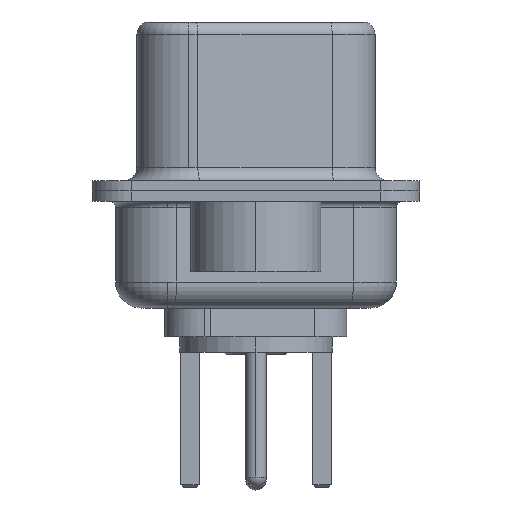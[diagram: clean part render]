
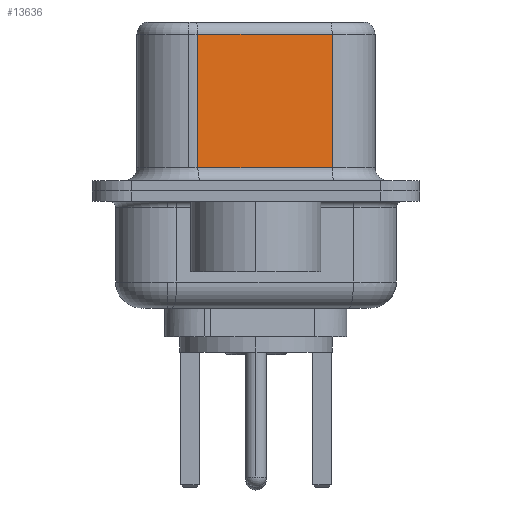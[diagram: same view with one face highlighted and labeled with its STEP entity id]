
A CAD part, left-side view. The second image highlights one B-rep face of the part: STEP entity #13636.
In plain terms, the highlighted planar face has unit normal (-0.985, -0.174, 0).
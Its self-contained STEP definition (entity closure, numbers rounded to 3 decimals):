
#1256 = VERTEX_POINT ( 'NONE', #13271 ) ;
#1541 = VECTOR ( 'NONE', #17890, 1000. ) ;
#1896 = DIRECTION ( 'NONE',  ( -0.174, 0.985, 0. ) ) ;
#2174 = EDGE_CURVE ( 'NONE', #6877, #3470, #17523, .T. ) ;
#2488 = EDGE_LOOP ( 'NONE', ( #5793, #9946, #18681, #13896 ) ) ;
#2517 = CARTESIAN_POINT ( 'NONE',  ( 4.565, -2.927, 6.02 ) ) ;
#3470 = VERTEX_POINT ( 'NONE', #10691 ) ;
#4288 = DIRECTION ( 'NONE',  ( 0., 0., -1. ) ) ;
#5793 = ORIENTED_EDGE ( 'NONE', *, *, #8785, .F. ) ;
#6603 = CARTESIAN_POINT ( 'NONE',  ( 4.565, -2.927, 6.02 ) ) ;
#6877 = VERTEX_POINT ( 'NONE', #15002 ) ;
#7883 = PLANE ( 'NONE',  #16694 ) ;
#7990 = LINE ( 'NONE', #17756, #15531 ) ;
#8785 = EDGE_CURVE ( 'NONE', #11197, #1256, #7990, .T. ) ;
#9412 = EDGE_CURVE ( 'NONE', #3470, #1256, #15061, .T. ) ;
#9946 = ORIENTED_EDGE ( 'NONE', *, *, #16346, .T. ) ;
#10691 = CARTESIAN_POINT ( 'NONE',  ( 3.655, 2.233, 0.9 ) ) ;
#10944 = DIRECTION ( 'NONE',  ( 0.985, 0.174, 0. ) ) ;
#11197 = VERTEX_POINT ( 'NONE', #2517 ) ;
#11621 = VECTOR ( 'NONE', #15582, 1000. ) ;
#12374 = FACE_OUTER_BOUND ( 'NONE', #2488, .T. ) ;
#13271 = CARTESIAN_POINT ( 'NONE',  ( 4.565, -2.927, 0.9 ) ) ;
#13485 = CARTESIAN_POINT ( 'NONE',  ( 3.655, 2.233, 6.52 ) ) ;
#13636 = ADVANCED_FACE ( 'NONE', ( #12374 ), #7883, .F. ) ;
#13896 = ORIENTED_EDGE ( 'NONE', *, *, #9412, .T. ) ;
#14994 = CARTESIAN_POINT ( 'NONE',  ( 4.565, -2.927, 0.9 ) ) ;
#15002 = CARTESIAN_POINT ( 'NONE',  ( 3.655, 2.233, 6.02 ) ) ;
#15061 = LINE ( 'NONE', #14994, #18496 ) ;
#15531 = VECTOR ( 'NONE', #4288, 1000. ) ;
#15582 = DIRECTION ( 'NONE',  ( -0.174, 0.985, 0. ) ) ;
#16346 = EDGE_CURVE ( 'NONE', #11197, #6877, #19481, .T. ) ;
#16417 = DIRECTION ( 'NONE',  ( 0.174, -0.985, 0. ) ) ;
#16694 = AXIS2_PLACEMENT_3D ( 'NONE', #18344, #10944, #1896 ) ;
#17523 = LINE ( 'NONE', #13485, #1541 ) ;
#17756 = CARTESIAN_POINT ( 'NONE',  ( 4.565, -2.927, 6.52 ) ) ;
#17890 = DIRECTION ( 'NONE',  ( 0., 0., -1. ) ) ;
#18344 = CARTESIAN_POINT ( 'NONE',  ( 4.565, -2.927, 6.52 ) ) ;
#18496 = VECTOR ( 'NONE', #16417, 1000. ) ;
#18681 = ORIENTED_EDGE ( 'NONE', *, *, #2174, .T. ) ;
#19481 = LINE ( 'NONE', #6603, #11621 ) ;
